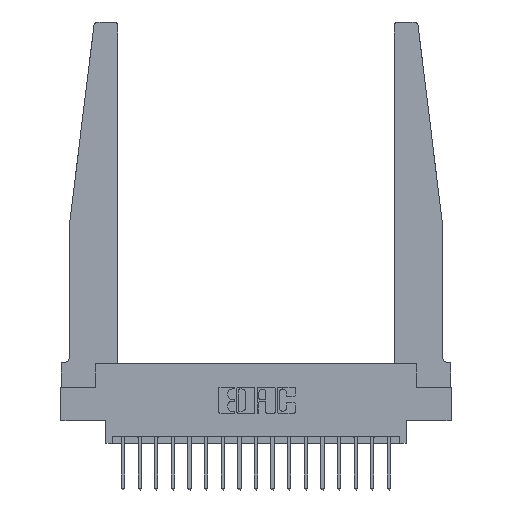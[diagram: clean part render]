
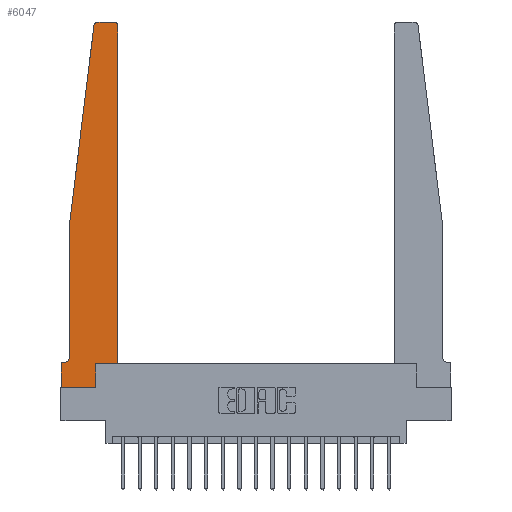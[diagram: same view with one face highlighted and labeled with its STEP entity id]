
A CAD part, top view. The second image highlights one B-rep face of the part: STEP entity #6047.
In plain terms, the highlighted planar face has unit normal (0, 0, 1).
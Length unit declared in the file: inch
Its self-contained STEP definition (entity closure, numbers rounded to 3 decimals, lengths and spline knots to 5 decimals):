
#350 = EDGE_CURVE ( 'NONE', #17635, #16318, #18981, .T. ) ;
#467 = DIRECTION ( 'NONE',  ( -1., 0., 0. ) ) ;
#536 = LINE ( 'NONE', #2139, #9376 ) ;
#600 = CARTESIAN_POINT ( 'NONE',  ( 0.395, 2.75, 0.37 ) ) ;
#644 = EDGE_CURVE ( 'NONE', #992, #2623, #17619, .T. ) ;
#876 = CARTESIAN_POINT ( 'NONE',  ( 0., 0., 0.37 ) ) ;
#950 = CARTESIAN_POINT ( 'NONE',  ( 0.2605, 0., 0.37 ) ) ;
#992 = VERTEX_POINT ( 'NONE', #12998 ) ;
#1329 = VERTEX_POINT ( 'NONE', #600 ) ;
#1470 = CIRCLE ( 'NONE', #19091, 0.05 ) ;
#1502 = DIRECTION ( 'NONE',  ( -0.122, -0.992, 0. ) ) ;
#1758 = DIRECTION ( 'NONE',  ( 0., 0., 1. ) ) ;
#1789 = VERTEX_POINT ( 'NONE', #19155 ) ;
#1972 = CARTESIAN_POINT ( 'NONE',  ( 0.015, 0.2375, 0.37 ) ) ;
#2139 = CARTESIAN_POINT ( 'NONE',  ( 0.425, 0.18, 0.37 ) ) ;
#2169 = VECTOR ( 'NONE', #16007, 39.37008 ) ;
#2283 = DIRECTION ( 'NONE',  ( 1., 0., 0. ) ) ;
#2623 = VERTEX_POINT ( 'NONE', #950 ) ;
#2937 = VECTOR ( 'NONE', #8714, 39.37008 ) ;
#3011 = LINE ( 'NONE', #12250, #18017 ) ;
#3079 = ORIENTED_EDGE ( 'NONE', *, *, #13735, .T. ) ;
#3295 = CARTESIAN_POINT ( 'NONE',  ( 0.015, 0.1875, 0.37 ) ) ;
#3367 = CARTESIAN_POINT ( 'NONE',  ( 0., 0.1875, 0.37 ) ) ;
#3418 = ORIENTED_EDGE ( 'NONE', *, *, #18020, .T. ) ;
#3481 = CARTESIAN_POINT ( 'NONE',  ( 0., 0.1875, 0.37 ) ) ;
#3547 = ORIENTED_EDGE ( 'NONE', *, *, #12946, .T. ) ;
#3549 = EDGE_CURVE ( 'NONE', #16318, #1329, #19279, .T. ) ;
#3955 = DIRECTION ( 'NONE',  ( 0., 1., 0. ) ) ;
#3991 = VECTOR ( 'NONE', #3955, 39.37008 ) ;
#5211 = CARTESIAN_POINT ( 'NONE',  ( 0.2605, 0.18, 0.37 ) ) ;
#5635 = ORIENTED_EDGE ( 'NONE', *, *, #14746, .T. ) ;
#6009 = AXIS2_PLACEMENT_3D ( 'NONE', #16025, #8140, #8039 ) ;
#6047 = ADVANCED_FACE ( 'NONE', ( #18515 ), #9310, .T. ) ;
#6394 = EDGE_CURVE ( 'NONE', #11804, #992, #16384, .T. ) ;
#6708 = EDGE_CURVE ( 'NONE', #9405, #17230, #3011, .T. ) ;
#6942 = VERTEX_POINT ( 'NONE', #3295 ) ;
#6949 = EDGE_CURVE ( 'NONE', #19165, #6942, #1470, .T. ) ;
#7077 = VERTEX_POINT ( 'NONE', #17731 ) ;
#7367 = LINE ( 'NONE', #18164, #14047 ) ;
#7871 = LINE ( 'NONE', #16759, #16955 ) ;
#7957 = DIRECTION ( 'NONE',  ( -1., 0., 0. ) ) ;
#8039 = DIRECTION ( 'NONE',  ( 1., 0., 0. ) ) ;
#8083 = AXIS2_PLACEMENT_3D ( 'NONE', #11740, #17826, #16303 ) ;
#8140 = DIRECTION ( 'NONE',  ( 0., 0., 1. ) ) ;
#8168 = VECTOR ( 'NONE', #2283, 39.37008 ) ;
#8714 = DIRECTION ( 'NONE',  ( 0., -1., 0. ) ) ;
#8945 = CARTESIAN_POINT ( 'NONE',  ( 0.065, 1.25, 0.37 ) ) ;
#9310 = PLANE ( 'NONE',  #14416 ) ;
#9369 = ORIENTED_EDGE ( 'NONE', *, *, #350, .T. ) ;
#9376 = VECTOR ( 'NONE', #14376, 39.37008 ) ;
#9405 = VERTEX_POINT ( 'NONE', #11998 ) ;
#9435 = DIRECTION ( 'NONE',  ( 0., 0., -1. ) ) ;
#9977 = CARTESIAN_POINT ( 'NONE',  ( 0.425, 0.18, 0.37 ) ) ;
#10079 = ORIENTED_EDGE ( 'NONE', *, *, #6708, .T. ) ;
#10102 = EDGE_CURVE ( 'NONE', #7077, #9405, #12085, .T. ) ;
#10219 = CARTESIAN_POINT ( 'NONE',  ( 0., 0., 0.37 ) ) ;
#11110 = CARTESIAN_POINT ( 'NONE',  ( 0.065, 0.2375, 0.37 ) ) ;
#11256 = ORIENTED_EDGE ( 'NONE', *, *, #6949, .T. ) ;
#11740 = CARTESIAN_POINT ( 'NONE',  ( 0.395, 2.72, 0.37 ) ) ;
#11804 = VERTEX_POINT ( 'NONE', #3481 ) ;
#11858 = EDGE_CURVE ( 'NONE', #17230, #19165, #13510, .T. ) ;
#11952 = EDGE_LOOP ( 'NONE', ( #5635, #18264, #10079, #14707, #11256, #3079, #16633, #19502, #3547, #3418, #9369, #13905 ) ) ;
#11998 = CARTESIAN_POINT ( 'NONE',  ( 0.24675, 2.72367, 0.37 ) ) ;
#12023 = CARTESIAN_POINT ( 'NONE',  ( 0.425, 0.18, 0.37 ) ) ;
#12085 = CIRCLE ( 'NONE', #6009, 0.03 ) ;
#12250 = CARTESIAN_POINT ( 'NONE',  ( 0.065, 1.25, 0.37 ) ) ;
#12946 = EDGE_CURVE ( 'NONE', #2623, #1789, #18930, .T. ) ;
#12998 = CARTESIAN_POINT ( 'NONE',  ( 0., 0., 0.37 ) ) ;
#13161 = DIRECTION ( 'NONE',  ( -1., 0., 0. ) ) ;
#13510 = LINE ( 'NONE', #17721, #15010 ) ;
#13735 = EDGE_CURVE ( 'NONE', #6942, #11804, #7367, .T. ) ;
#13905 = ORIENTED_EDGE ( 'NONE', *, *, #3549, .T. ) ;
#14047 = VECTOR ( 'NONE', #13161, 39.37008 ) ;
#14376 = DIRECTION ( 'NONE',  ( 1., 0., 0. ) ) ;
#14416 = AXIS2_PLACEMENT_3D ( 'NONE', #3367, #1758, #15179 ) ;
#14707 = ORIENTED_EDGE ( 'NONE', *, *, #11858, .T. ) ;
#14746 = EDGE_CURVE ( 'NONE', #1329, #7077, #7871, .T. ) ;
#15010 = VECTOR ( 'NONE', #16403, 39.37008 ) ;
#15179 = DIRECTION ( 'NONE',  ( 1., 0., 0. ) ) ;
#15536 = CARTESIAN_POINT ( 'NONE',  ( 0.425, 2.72, 0.37 ) ) ;
#16007 = DIRECTION ( 'NONE',  ( 0., 1., 0. ) ) ;
#16025 = CARTESIAN_POINT ( 'NONE',  ( 0.27653, 2.72, 0.37 ) ) ;
#16303 = DIRECTION ( 'NONE',  ( 1., 0., 0. ) ) ;
#16318 = VERTEX_POINT ( 'NONE', #15536 ) ;
#16384 = LINE ( 'NONE', #10219, #2937 ) ;
#16403 = DIRECTION ( 'NONE',  ( 0., -1., 0. ) ) ;
#16633 = ORIENTED_EDGE ( 'NONE', *, *, #6394, .T. ) ;
#16759 = CARTESIAN_POINT ( 'NONE',  ( 0.25, 2.75, 0.37 ) ) ;
#16955 = VECTOR ( 'NONE', #7957, 39.37008 ) ;
#17230 = VERTEX_POINT ( 'NONE', #8945 ) ;
#17619 = LINE ( 'NONE', #876, #8168 ) ;
#17635 = VERTEX_POINT ( 'NONE', #12023 ) ;
#17721 = CARTESIAN_POINT ( 'NONE',  ( 0.065, 1.25, 0.37 ) ) ;
#17731 = CARTESIAN_POINT ( 'NONE',  ( 0.27653, 2.75, 0.37 ) ) ;
#17826 = DIRECTION ( 'NONE',  ( 0., 0., 1. ) ) ;
#18017 = VECTOR ( 'NONE', #1502, 39.37008 ) ;
#18020 = EDGE_CURVE ( 'NONE', #1789, #17635, #536, .T. ) ;
#18164 = CARTESIAN_POINT ( 'NONE',  ( 0.065, 0.1875, 0.37 ) ) ;
#18264 = ORIENTED_EDGE ( 'NONE', *, *, #10102, .T. ) ;
#18515 = FACE_OUTER_BOUND ( 'NONE', #11952, .T. ) ;
#18930 = LINE ( 'NONE', #5211, #2169 ) ;
#18981 = LINE ( 'NONE', #9977, #3991 ) ;
#19091 = AXIS2_PLACEMENT_3D ( 'NONE', #1972, #9435, #467 ) ;
#19155 = CARTESIAN_POINT ( 'NONE',  ( 0.2605, 0.18, 0.37 ) ) ;
#19165 = VERTEX_POINT ( 'NONE', #11110 ) ;
#19279 = CIRCLE ( 'NONE', #8083, 0.03 ) ;
#19502 = ORIENTED_EDGE ( 'NONE', *, *, #644, .T. ) ;
